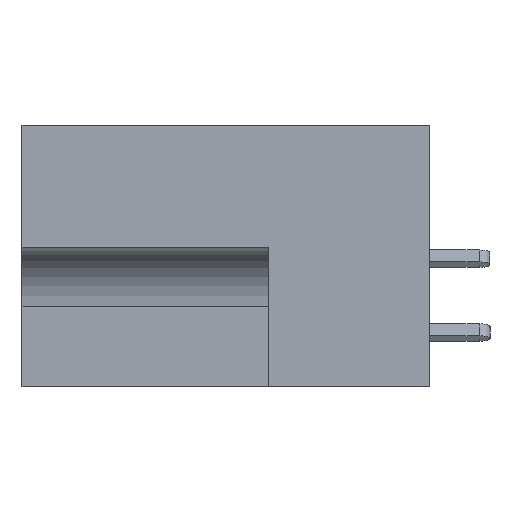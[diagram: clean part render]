
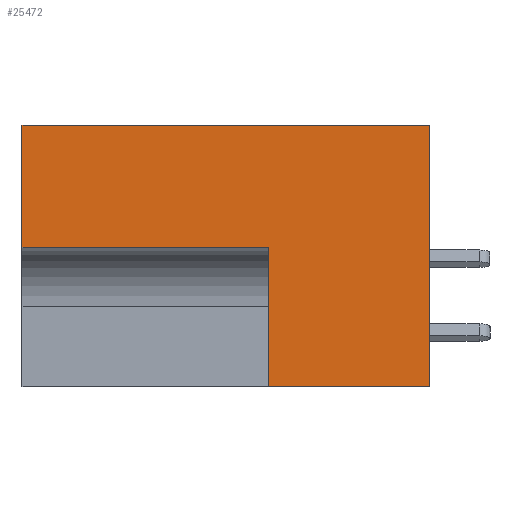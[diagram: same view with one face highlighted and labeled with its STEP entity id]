
A CAD part, left-side view. The second image highlights one B-rep face of the part: STEP entity #25472.
In plain terms, the highlighted planar face has unit normal (-1, 0, 0).
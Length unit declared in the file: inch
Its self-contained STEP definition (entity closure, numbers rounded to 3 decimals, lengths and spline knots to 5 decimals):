
#648 = VERTEX_POINT ( 'NONE', #8295 ) ;
#821 = LINE ( 'NONE', #6371, #12069 ) ;
#884 = ORIENTED_EDGE ( 'NONE', *, *, #27686, .F. ) ;
#890 = CARTESIAN_POINT ( 'NONE',  ( 0., 0.328, -0.531 ) ) ;
#1155 = VERTEX_POINT ( 'NONE', #25490 ) ;
#1636 = ORIENTED_EDGE ( 'NONE', *, *, #21281, .T. ) ;
#1647 = VERTEX_POINT ( 'NONE', #22532 ) ;
#1877 = LINE ( 'NONE', #16082, #5639 ) ;
#1910 = LINE ( 'NONE', #18904, #11833 ) ;
#4323 = DIRECTION ( 'NONE',  ( 0., -1., 0. ) ) ;
#5639 = VECTOR ( 'NONE', #24474, 39.37008 ) ;
#5887 = DIRECTION ( 'NONE',  ( 0., 0., 1. ) ) ;
#6162 = EDGE_CURVE ( 'NONE', #9941, #648, #821, .T. ) ;
#6371 = CARTESIAN_POINT ( 'NONE',  ( 0., 0., 0. ) ) ;
#6693 = CARTESIAN_POINT ( 'NONE',  ( 0., 0., -0.531 ) ) ;
#7810 = VECTOR ( 'NONE', #16115, 39.37008 ) ;
#8205 = FACE_OUTER_BOUND ( 'NONE', #21147, .T. ) ;
#8295 = CARTESIAN_POINT ( 'NONE',  ( 0., 0., 0. ) ) ;
#8629 = ORIENTED_EDGE ( 'NONE', *, *, #25887, .F. ) ;
#8862 = LINE ( 'NONE', #17130, #10588 ) ;
#9516 = ORIENTED_EDGE ( 'NONE', *, *, #6162, .T. ) ;
#9941 = VERTEX_POINT ( 'NONE', #6693 ) ;
#10588 = VECTOR ( 'NONE', #19405, 39.37008 ) ;
#10981 = ORIENTED_EDGE ( 'NONE', *, *, #20406, .F. ) ;
#11292 = CARTESIAN_POINT ( 'NONE',  ( 0., 0.453, 0. ) ) ;
#11833 = VECTOR ( 'NONE', #5887, 39.37008 ) ;
#12069 = VECTOR ( 'NONE', #12754, 39.37008 ) ;
#12754 = DIRECTION ( 'NONE',  ( 0., 0., 1. ) ) ;
#16082 = CARTESIAN_POINT ( 'NONE',  ( 0., 0.453, -0.531 ) ) ;
#16115 = DIRECTION ( 'NONE',  ( 0., 0., 1. ) ) ;
#16152 = EDGE_CURVE ( 'NONE', #1155, #1647, #25190, .T. ) ;
#17130 = CARTESIAN_POINT ( 'NONE',  ( 0., 0.328, -0.248 ) ) ;
#17822 = CARTESIAN_POINT ( 'NONE',  ( 0., 0.453, 0. ) ) ;
#18904 = CARTESIAN_POINT ( 'NONE',  ( 0., 0.828, 0. ) ) ;
#18965 = VECTOR ( 'NONE', #4323, 39.37008 ) ;
#19405 = DIRECTION ( 'NONE',  ( 0., 1., 0. ) ) ;
#20406 = EDGE_CURVE ( 'NONE', #25427, #648, #21009, .T. ) ;
#21009 = LINE ( 'NONE', #11292, #18965 ) ;
#21147 = EDGE_LOOP ( 'NONE', ( #884, #8629, #27367, #1636, #9516, #10981 ) ) ;
#21281 = EDGE_CURVE ( 'NONE', #1155, #9941, #1877, .T. ) ;
#22532 = CARTESIAN_POINT ( 'NONE',  ( 0., 0.328, -0.248 ) ) ;
#22863 = VERTEX_POINT ( 'NONE', #26384 ) ;
#24225 = CARTESIAN_POINT ( 'NONE',  ( 0., 0.828, 0. ) ) ;
#24311 = PLANE ( 'NONE',  #26357 ) ;
#24406 = DIRECTION ( 'NONE',  ( 0., 0., -1. ) ) ;
#24474 = DIRECTION ( 'NONE',  ( 0., -1., 0. ) ) ;
#25190 = LINE ( 'NONE', #890, #7810 ) ;
#25427 = VERTEX_POINT ( 'NONE', #24225 ) ;
#25472 = ADVANCED_FACE ( 'NONE', ( #8205 ), #24311, .F. ) ;
#25490 = CARTESIAN_POINT ( 'NONE',  ( 0., 0.328, -0.531 ) ) ;
#25887 = EDGE_CURVE ( 'NONE', #1647, #22863, #8862, .T. ) ;
#26357 = AXIS2_PLACEMENT_3D ( 'NONE', #17822, #26606, #24406 ) ;
#26384 = CARTESIAN_POINT ( 'NONE',  ( 0., 0.828, -0.248 ) ) ;
#26606 = DIRECTION ( 'NONE',  ( 1., 0., 0. ) ) ;
#27367 = ORIENTED_EDGE ( 'NONE', *, *, #16152, .F. ) ;
#27686 = EDGE_CURVE ( 'NONE', #22863, #25427, #1910, .T. ) ;
